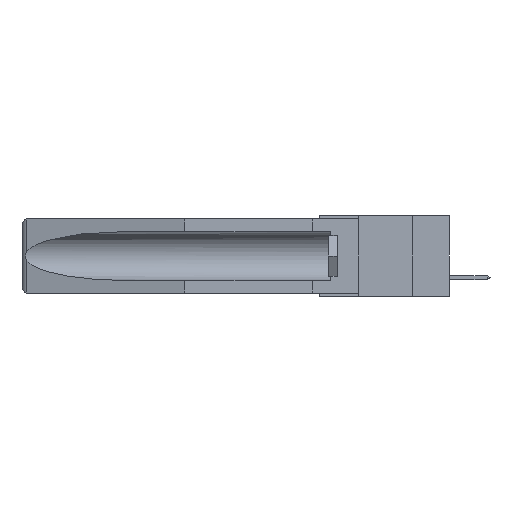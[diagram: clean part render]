
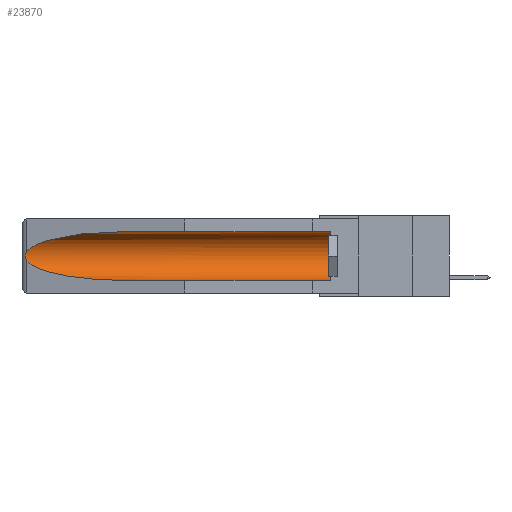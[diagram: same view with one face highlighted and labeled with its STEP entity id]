
A CAD part, left-side view. The second image highlights one B-rep face of the part: STEP entity #23870.
In plain terms, the highlighted cylindrical face has radius 2.857 mm (diameter 5.715 mm), a partial arc.
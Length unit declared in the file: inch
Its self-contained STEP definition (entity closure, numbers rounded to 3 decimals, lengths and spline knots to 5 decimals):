
#75 = CARTESIAN_POINT ( 'NONE',  ( 0.26537, 1.52718, -0.19328 ) ) ;
#1237 = DIRECTION ( 'NONE',  ( 0., 0., 1. ) ) ;
#1449 = CARTESIAN_POINT ( 'NONE',  ( 0.155, -0.30754, -0.1715 ) ) ;
#1623 = ORIENTED_EDGE ( 'NONE', *, *, #29005, .T. ) ;
#2485 = EDGE_CURVE ( 'NONE', #4815, #26023, #9703, .T. ) ;
#2890 = ORIENTED_EDGE ( 'NONE', *, *, #22875, .T. ) ;
#3018 = CARTESIAN_POINT ( 'NONE',  ( 0.25451, 1.48313, -0.24835 ) ) ;
#3286 = CARTESIAN_POINT ( 'NONE',  ( 0.26537, 1.52718, -0.14972 ) ) ;
#3893 = CARTESIAN_POINT ( 'NONE',  ( 0.2673, 1.5327, -0.16383 ) ) ;
#4124 = CARTESIAN_POINT ( 'NONE',  ( 0.26537, 1.52718, -0.19328 ) ) ;
#4815 = VERTEX_POINT ( 'NONE', #28547 ) ;
#5841 = VERTEX_POINT ( 'NONE', #27688 ) ;
#5990 = ORIENTED_EDGE ( 'NONE', *, *, #8369, .F. ) ;
#8316 = CARTESIAN_POINT ( 'NONE',  ( 0.155, 1.07973, -0.059 ) ) ;
#8369 = EDGE_CURVE ( 'NONE', #5841, #28804, #32623, .T. ) ;
#9703 =( BOUNDED_CURVE ( )  B_SPLINE_CURVE ( 3, ( #8316, #23390, #16074, #3286 ),
 .UNSPECIFIED., .F., .F. ) 
 B_SPLINE_CURVE_WITH_KNOTS ( ( 4, 4 ),
 ( 4.71239, 6.08839 ),
 .UNSPECIFIED. ) 
 CURVE ( )  GEOMETRIC_REPRESENTATION_ITEM ( )  RATIONAL_B_SPLINE_CURVE ( ( 1., 0.848, 0.848, 1. ) ) 
 REPRESENTATION_ITEM ( '' )  );
#10130 = DIRECTION ( 'NONE',  ( 0., 0., 1. ) ) ;
#10514 = CARTESIAN_POINT ( 'NONE',  ( 0.155, -0.30754, -0.059 ) ) ;
#10877 = CARTESIAN_POINT ( 'NONE',  ( 0.26597, 1.52961, -0.15275 ) ) ;
#11391 = EDGE_LOOP ( 'NONE', ( #31918, #14017, #27392, #5990, #1623, #2890 ) ) ;
#11632 = LINE ( 'NONE', #10514, #23684 ) ;
#12118 = VECTOR ( 'NONE', #18422, 39.37008 ) ;
#13042 = CARTESIAN_POINT ( 'NONE',  ( 0.155, 0.126, -0.1715 ) ) ;
#13155 = CARTESIAN_POINT ( 'NONE',  ( 0.26537, 1.52718, -0.19328 ) ) ;
#13257 = CARTESIAN_POINT ( 'NONE',  ( 0.155, 1.07973, -0.284 ) ) ;
#13790 = CARTESIAN_POINT ( 'NONE',  ( 0.26537, 1.52718, -0.14972 ) ) ;
#14017 = ORIENTED_EDGE ( 'NONE', *, *, #20620, .T. ) ;
#14064 = AXIS2_PLACEMENT_3D ( 'NONE', #1449, #32375, #1237 ) ;
#14863 = CARTESIAN_POINT ( 'NONE',  ( 0.155, 0.126, -0.059 ) ) ;
#15558 = CIRCLE ( 'NONE', #19491, 0.1125 ) ;
#15839 = CARTESIAN_POINT ( 'NONE',  ( 0.21114, 1.30732, -0.284 ) ) ;
#15869 = CARTESIAN_POINT ( 'NONE',  ( 0.155, -0.30754, -0.284 ) ) ;
#16074 = CARTESIAN_POINT ( 'NONE',  ( 0.25451, 1.48313, -0.09465 ) ) ;
#18364 = FACE_OUTER_BOUND ( 'NONE', #11391, .T. ) ;
#18422 = DIRECTION ( 'NONE',  ( 0., 1., 0. ) ) ;
#19491 = AXIS2_PLACEMENT_3D ( 'NONE', #13042, #25853, #10130 ) ;
#19565 =( BOUNDED_CURVE ( )  B_SPLINE_CURVE ( 3, ( #13155, #3018, #15839, #13257 ),
 .UNSPECIFIED., .F., .F. ) 
 B_SPLINE_CURVE_WITH_KNOTS ( ( 4, 4 ),
 ( 0.1948, 1.5708 ),
 .UNSPECIFIED. ) 
 CURVE ( )  GEOMETRIC_REPRESENTATION_ITEM ( )  RATIONAL_B_SPLINE_CURVE ( ( 1., 0.848, 0.848, 1. ) ) 
 REPRESENTATION_ITEM ( '' )  );
#19859 = CARTESIAN_POINT ( 'NONE',  ( 0.155, 1.07973, -0.284 ) ) ;
#20620 = EDGE_CURVE ( 'NONE', #26023, #30950, #22044, .T. ) ;
#21841 = CARTESIAN_POINT ( 'NONE',  ( 0.26597, 1.5296, -0.19026 ) ) ;
#22044 = B_SPLINE_CURVE_WITH_KNOTS ( 'NONE', 3,
 ( #13790, #10877, #24576, #3893, #24462, #27304, #32215, #24228, #21841, #4124 ),
 .UNSPECIFIED., .F., .F.,
 ( 4, 2, 2, 2, 4 ),
 ( 0., 0.00029, 0.00058, 0.00087, 0.00117 ),
 .UNSPECIFIED. ) ;
#22875 = EDGE_CURVE ( 'NONE', #25517, #4815, #11632, .T. ) ;
#23390 = CARTESIAN_POINT ( 'NONE',  ( 0.21114, 1.30732, -0.059 ) ) ;
#23590 = CARTESIAN_POINT ( 'NONE',  ( 0.26537, 1.52718, -0.14972 ) ) ;
#23684 = VECTOR ( 'NONE', #25683, 39.37008 ) ;
#23870 = ADVANCED_FACE ( 'NONE', ( #18364 ), #29276, .F. ) ;
#24228 = CARTESIAN_POINT ( 'NONE',  ( 0.26655, 1.53094, -0.18657 ) ) ;
#24462 = CARTESIAN_POINT ( 'NONE',  ( 0.2675, 1.53308, -0.16763 ) ) ;
#24576 = CARTESIAN_POINT ( 'NONE',  ( 0.26654, 1.53092, -0.15636 ) ) ;
#25517 = VERTEX_POINT ( 'NONE', #14863 ) ;
#25683 = DIRECTION ( 'NONE',  ( 0., 1., 0. ) ) ;
#25853 = DIRECTION ( 'NONE',  ( 0., -1., 0. ) ) ;
#26023 = VERTEX_POINT ( 'NONE', #23590 ) ;
#27304 = CARTESIAN_POINT ( 'NONE',  ( 0.2675, 1.53308, -0.17534 ) ) ;
#27392 = ORIENTED_EDGE ( 'NONE', *, *, #27405, .T. ) ;
#27405 = EDGE_CURVE ( 'NONE', #30950, #28804, #19565, .T. ) ;
#27688 = CARTESIAN_POINT ( 'NONE',  ( 0.155, 0.126, -0.284 ) ) ;
#28547 = CARTESIAN_POINT ( 'NONE',  ( 0.155, 1.07973, -0.059 ) ) ;
#28804 = VERTEX_POINT ( 'NONE', #19859 ) ;
#29005 = EDGE_CURVE ( 'NONE', #5841, #25517, #15558, .T. ) ;
#29276 = CYLINDRICAL_SURFACE ( 'NONE', #14064, 0.1125 ) ;
#30950 = VERTEX_POINT ( 'NONE', #75 ) ;
#31918 = ORIENTED_EDGE ( 'NONE', *, *, #2485, .T. ) ;
#32215 = CARTESIAN_POINT ( 'NONE',  ( 0.2673, 1.53269, -0.17917 ) ) ;
#32375 = DIRECTION ( 'NONE',  ( 0., 1., 0. ) ) ;
#32623 = LINE ( 'NONE', #15869, #12118 ) ;
